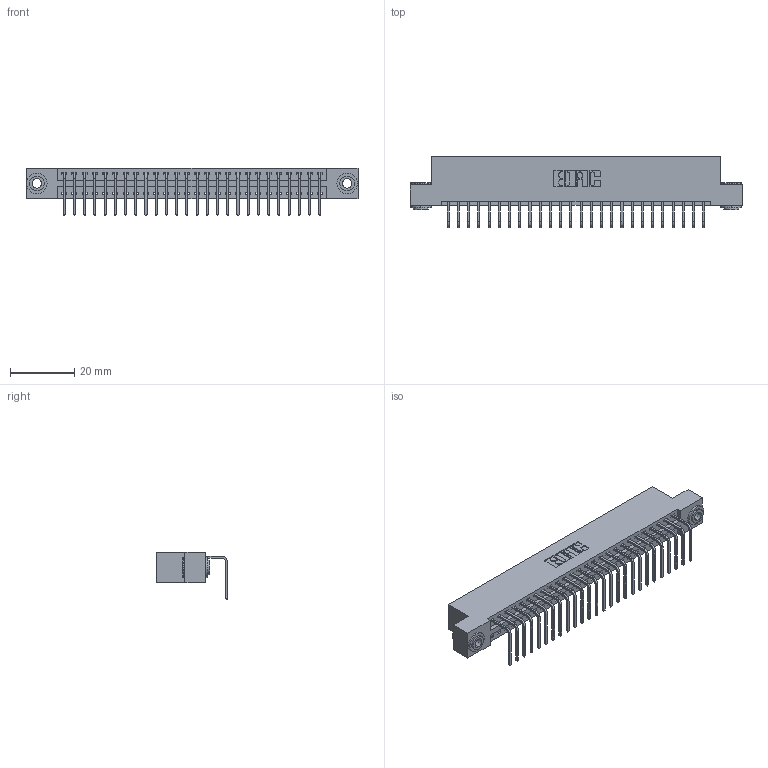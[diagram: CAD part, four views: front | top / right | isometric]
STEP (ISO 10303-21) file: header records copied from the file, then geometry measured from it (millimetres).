
FILE_DESCRIPTION (( 'STEP AP203' ), '1' );
FILE_NAME ('346-026-558-103.STEP', '2022-05-06T03:19:52', ( '' ), ( '' ), 'SwSTEP 2.0', 'SolidWorks 2020', '' );
FILE_SCHEMA (( 'CONFIG_CONTROL_DESIGN' ));
Length unit declared in the file: inch
Products named in the file (4): 345-292-001_558 Tail - 2; 346-026-558-103; 346 Part_Flush Mounting Lugs - 0.156 Dia-TH; 345-250-002_345-250-002-102
Assembly tree (29 placements, depth 2):
  346-026-558-103
    346 Part_Flush Mounting Lugs - 0.156 Dia-TH
    345-292-001_558 Tail - 2  x26
    345-250-002_345-250-002-102  x2
Bounding box: 103.12 x 22.16 x 14.73 mm (x, y, z)
Volume: 9848.9 mm3; surface area: 12905.5 mm2
Topology: 29 solids, 29 shells, 1734 faces, 5173 edges, 3410 vertices
Faces by surface type: plane 1192, cylinder 534, cone 8
Entity records: 19440 total; most frequent: CARTESIAN_POINT 3319, ORIENTED_EDGE 3270, DIRECTION 2977, EDGE_CURVE 1635, LINE 1375, VECTOR 1375, VERTEX_POINT 1086, AXIS2_PLACEMENT_3D 801
